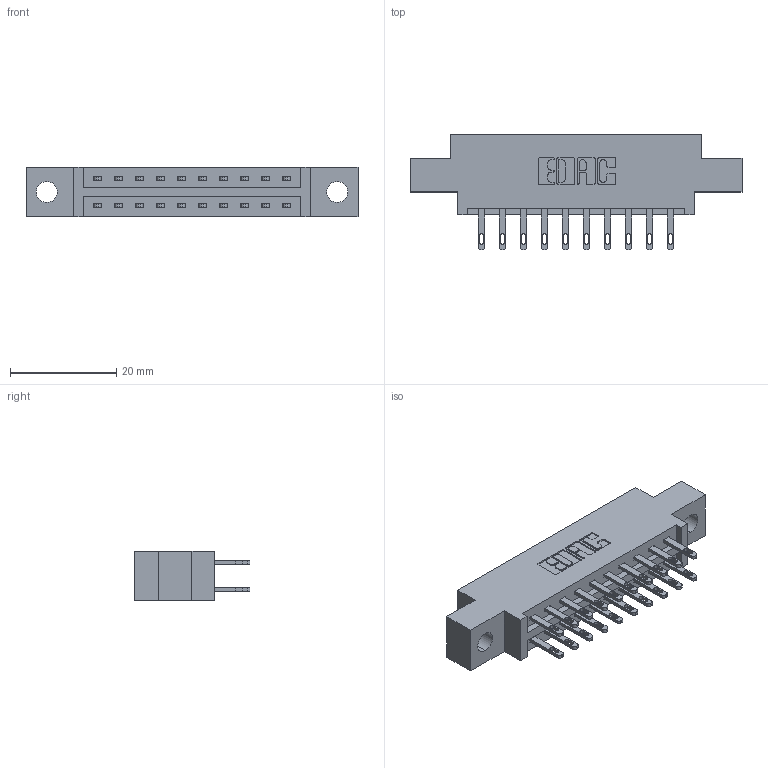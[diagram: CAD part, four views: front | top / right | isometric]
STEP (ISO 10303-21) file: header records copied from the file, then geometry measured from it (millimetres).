
FILE_DESCRIPTION (( 'STEP AP203' ), '1' );
FILE_NAME ('337-020-500-804.STEP', '2018-08-05T08:04:24', ( '' ), ( '' ), 'SwSTEP 2.0', 'SolidWorks 2016', '' );
FILE_SCHEMA (( 'CONFIG_CONTROL_DESIGN' ));
Length unit declared in the file: inch
Products named in the file (3): 345-292-001_345-293-100; 337-020-500-804; 337 Part_0.170 Offset - 0.156 Dia-TH
Assembly tree (21 placements, depth 2):
  337-020-500-804
    337 Part_0.170 Offset - 0.156 Dia-TH
    345-292-001_345-293-100  x20
Bounding box: 62.64 x 21.85 x 9.4 mm (x, y, z)
Volume: 6030.9 mm3; surface area: 6634.3 mm2
Topology: 21 solids, 21 shells, 1118 faces, 3383 edges, 2254 vertices
Faces by surface type: plane 714, cylinder 404
Entity records: 11957 total; most frequent: CARTESIAN_POINT 2042, ORIENTED_EDGE 1978, DIRECTION 1797, EDGE_CURVE 989, LINE 857, VECTOR 857, VERTEX_POINT 658, AXIS2_PLACEMENT_3D 470
